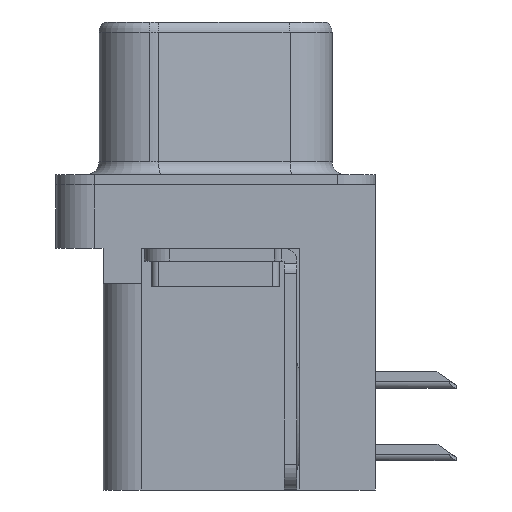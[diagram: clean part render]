
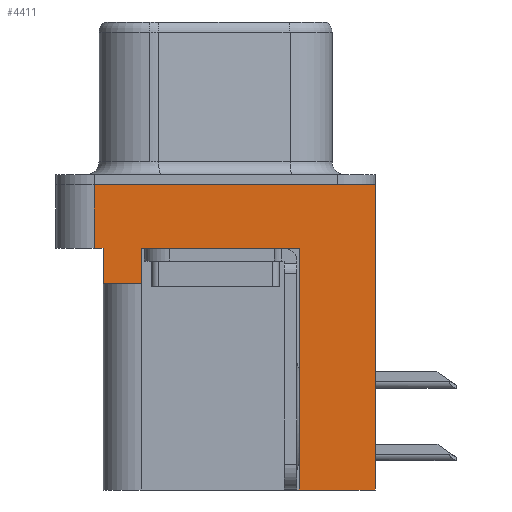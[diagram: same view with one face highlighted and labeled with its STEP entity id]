
A CAD part, left-side view. The second image highlights one B-rep face of the part: STEP entity #4411.
In plain terms, the highlighted planar face has unit normal (-1, 0, 0).
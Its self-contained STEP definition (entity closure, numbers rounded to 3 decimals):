
#208 = DIRECTION ( 'NONE',  ( -1., 0., 0. ) ) ;
#246 = ORIENTED_EDGE ( 'NONE', *, *, #4984, .F. ) ;
#344 = LINE ( 'NONE', #17606, #573 ) ;
#573 = VECTOR ( 'NONE', #10967, 1000. ) ;
#634 = DIRECTION ( 'NONE',  ( 0., 0., 1. ) ) ;
#965 = LINE ( 'NONE', #12559, #15442 ) ;
#1446 = VECTOR ( 'NONE', #17236, 1000. ) ;
#1604 = VERTEX_POINT ( 'NONE', #12639 ) ;
#1618 = DIRECTION ( 'NONE',  ( 0., 0., 1. ) ) ;
#1942 = CARTESIAN_POINT ( 'NONE',  ( -2.91, -3.295, -12. ) ) ;
#2057 = CARTESIAN_POINT ( 'NONE',  ( -2.91, 4.775, 0. ) ) ;
#2081 = LINE ( 'NONE', #1942, #12581 ) ;
#2342 = ORIENTED_EDGE ( 'NONE', *, *, #2672, .F. ) ;
#2386 = DIRECTION ( 'NONE',  ( 0., -1., 0. ) ) ;
#2672 = EDGE_CURVE ( 'NONE', #14488, #8192, #14396, .T. ) ;
#3070 = ORIENTED_EDGE ( 'NONE', *, *, #4506, .T. ) ;
#3163 = CARTESIAN_POINT ( 'NONE',  ( -2.91, 2.895, -2.5 ) ) ;
#3187 = CARTESIAN_POINT ( 'NONE',  ( -2.91, 4.775, -2.5 ) ) ;
#3325 = VERTEX_POINT ( 'NONE', #16908 ) ;
#3964 = CARTESIAN_POINT ( 'NONE',  ( -2.91, -6.275, -2.5 ) ) ;
#3996 = CARTESIAN_POINT ( 'NONE',  ( -2.91, 4.425, -3.9 ) ) ;
#4171 = VECTOR ( 'NONE', #7210, 1000. ) ;
#4236 = EDGE_CURVE ( 'NONE', #8192, #5350, #16191, .T. ) ;
#4263 = VERTEX_POINT ( 'NONE', #2057 ) ;
#4411 = ADVANCED_FACE ( 'NONE', ( #8010 ), #11411, .T. ) ;
#4506 = EDGE_CURVE ( 'NONE', #14488, #10208, #344, .T. ) ;
#4584 = CARTESIAN_POINT ( 'NONE',  ( -2.91, -6.275, -12. ) ) ;
#4593 = CARTESIAN_POINT ( 'NONE',  ( -2.91, -3.295, -12. ) ) ;
#4876 = LINE ( 'NONE', #3964, #5107 ) ;
#4984 = EDGE_CURVE ( 'NONE', #1604, #3325, #12859, .T. ) ;
#5039 = AXIS2_PLACEMENT_3D ( 'NONE', #14039, #208, #17127 ) ;
#5107 = VECTOR ( 'NONE', #2386, 1000. ) ;
#5350 = VERTEX_POINT ( 'NONE', #14407 ) ;
#6004 = EDGE_CURVE ( 'NONE', #4263, #10370, #18121, .T. ) ;
#6799 = EDGE_LOOP ( 'NONE', ( #18112, #10949, #12378, #9330, #2342, #3070, #11661, #246, #12215, #14078 ) ) ;
#6881 = CARTESIAN_POINT ( 'NONE',  ( -2.91, -6.275, 0. ) ) ;
#7191 = DIRECTION ( 'NONE',  ( 0., 1., 0. ) ) ;
#7210 = DIRECTION ( 'NONE',  ( 0., 0., 1. ) ) ;
#7359 = VECTOR ( 'NONE', #634, 1000. ) ;
#8010 = FACE_OUTER_BOUND ( 'NONE', #6799, .T. ) ;
#8192 = VERTEX_POINT ( 'NONE', #3996 ) ;
#8254 = CARTESIAN_POINT ( 'NONE',  ( -2.91, -6.275, -2.5 ) ) ;
#9049 = DIRECTION ( 'NONE',  ( 0., -1., 0. ) ) ;
#9330 = ORIENTED_EDGE ( 'NONE', *, *, #4236, .F. ) ;
#9916 = VERTEX_POINT ( 'NONE', #4584 ) ;
#10052 = LINE ( 'NONE', #14245, #4171 ) ;
#10208 = VERTEX_POINT ( 'NONE', #3163 ) ;
#10370 = VERTEX_POINT ( 'NONE', #11301 ) ;
#10949 = ORIENTED_EDGE ( 'NONE', *, *, #17218, .F. ) ;
#10967 = DIRECTION ( 'NONE',  ( 0., 0., 1. ) ) ;
#11054 = VECTOR ( 'NONE', #16728, 1000. ) ;
#11301 = CARTESIAN_POINT ( 'NONE',  ( -2.91, -6.275, 0. ) ) ;
#11411 = PLANE ( 'NONE',  #5039 ) ;
#11457 = VECTOR ( 'NONE', #9049, 1000. ) ;
#11641 = CARTESIAN_POINT ( 'NONE',  ( -2.91, 2.895, -3.9 ) ) ;
#11661 = ORIENTED_EDGE ( 'NONE', *, *, #17535, .T. ) ;
#12063 = EDGE_CURVE ( 'NONE', #9916, #10370, #10052, .T. ) ;
#12138 = VERTEX_POINT ( 'NONE', #3187 ) ;
#12215 = ORIENTED_EDGE ( 'NONE', *, *, #17290, .F. ) ;
#12378 = ORIENTED_EDGE ( 'NONE', *, *, #18184, .T. ) ;
#12559 = CARTESIAN_POINT ( 'NONE',  ( -2.91, 4.775, -2.5 ) ) ;
#12581 = VECTOR ( 'NONE', #17247, 1000. ) ;
#12639 = CARTESIAN_POINT ( 'NONE',  ( -2.91, -3.295, -12. ) ) ;
#12859 = LINE ( 'NONE', #4593, #1446 ) ;
#12874 = CARTESIAN_POINT ( 'NONE',  ( -2.91, 4.425, -3.9 ) ) ;
#14039 = CARTESIAN_POINT ( 'NONE',  ( -2.91, -6.275, -2.5 ) ) ;
#14078 = ORIENTED_EDGE ( 'NONE', *, *, #12063, .T. ) ;
#14245 = CARTESIAN_POINT ( 'NONE',  ( -2.91, -6.275, -2.5 ) ) ;
#14396 = LINE ( 'NONE', #12874, #14611 ) ;
#14407 = CARTESIAN_POINT ( 'NONE',  ( -2.91, 4.425, -2.5 ) ) ;
#14488 = VERTEX_POINT ( 'NONE', #11641 ) ;
#14611 = VECTOR ( 'NONE', #7191, 1000. ) ;
#15241 = LINE ( 'NONE', #8254, #11457 ) ;
#15442 = VECTOR ( 'NONE', #1618, 1000. ) ;
#16041 = CARTESIAN_POINT ( 'NONE',  ( -2.91, 4.425, -3.9 ) ) ;
#16191 = LINE ( 'NONE', #16041, #7359 ) ;
#16728 = DIRECTION ( 'NONE',  ( 0., -1., 0. ) ) ;
#16908 = CARTESIAN_POINT ( 'NONE',  ( -2.91, -3.295, -2.5 ) ) ;
#17127 = DIRECTION ( 'NONE',  ( 0., 0., 1. ) ) ;
#17218 = EDGE_CURVE ( 'NONE', #12138, #4263, #965, .T. ) ;
#17236 = DIRECTION ( 'NONE',  ( 0., 0., 1. ) ) ;
#17247 = DIRECTION ( 'NONE',  ( 0., 1., 0. ) ) ;
#17290 = EDGE_CURVE ( 'NONE', #9916, #1604, #2081, .T. ) ;
#17535 = EDGE_CURVE ( 'NONE', #10208, #3325, #15241, .T. ) ;
#17606 = CARTESIAN_POINT ( 'NONE',  ( -2.91, 2.895, -3.9 ) ) ;
#18112 = ORIENTED_EDGE ( 'NONE', *, *, #6004, .F. ) ;
#18121 = LINE ( 'NONE', #6881, #11054 ) ;
#18184 = EDGE_CURVE ( 'NONE', #12138, #5350, #4876, .T. ) ;
